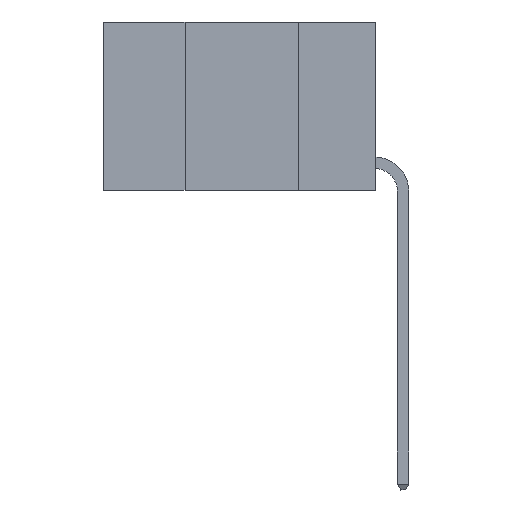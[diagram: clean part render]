
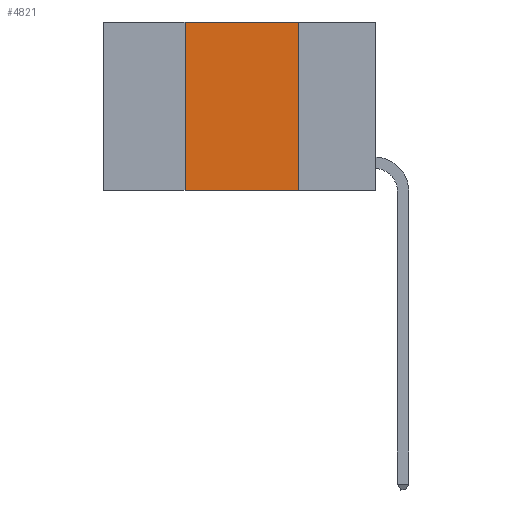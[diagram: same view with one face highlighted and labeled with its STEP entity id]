
A CAD part, left-side view. The second image highlights one B-rep face of the part: STEP entity #4821.
In plain terms, the highlighted planar face has unit normal (-1, 0, 0).
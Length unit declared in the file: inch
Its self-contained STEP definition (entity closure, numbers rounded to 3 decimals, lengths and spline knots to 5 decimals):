
#1 = DIRECTION ( 'NONE',  ( 0., 0., 1. ) ) ;
#532 = VECTOR ( 'NONE', #12277, 39.37008 ) ;
#628 = ORIENTED_EDGE ( 'NONE', *, *, #4704, .F. ) ;
#1104 = DIRECTION ( 'NONE',  ( 0., -1., 0. ) ) ;
#1490 = VERTEX_POINT ( 'NONE', #5422 ) ;
#1825 = VERTEX_POINT ( 'NONE', #3805 ) ;
#1961 = VERTEX_POINT ( 'NONE', #15304 ) ;
#2581 = ORIENTED_EDGE ( 'NONE', *, *, #4188, .F. ) ;
#2772 = DIRECTION ( 'NONE',  ( 1., 0., 0. ) ) ;
#3540 = CARTESIAN_POINT ( 'NONE',  ( 0., 0.17, 0. ) ) ;
#3805 = CARTESIAN_POINT ( 'NONE',  ( 0., 0.42, 0. ) ) ;
#4188 = EDGE_CURVE ( 'NONE', #1825, #1961, #5525, .T. ) ;
#4704 = EDGE_CURVE ( 'NONE', #1961, #10951, #6226, .T. ) ;
#4821 = ADVANCED_FACE ( 'NONE', ( #10494 ), #7730, .F. ) ;
#5422 = CARTESIAN_POINT ( 'NONE',  ( 0., 0.42, -0.37 ) ) ;
#5525 = LINE ( 'NONE', #9837, #532 ) ;
#6067 = CARTESIAN_POINT ( 'NONE',  ( 0., 0.6, -0.37 ) ) ;
#6226 = LINE ( 'NONE', #3540, #11155 ) ;
#7207 = VECTOR ( 'NONE', #1104, 39.37008 ) ;
#7730 = PLANE ( 'NONE',  #14382 ) ;
#8379 = ORIENTED_EDGE ( 'NONE', *, *, #8780, .T. ) ;
#8780 = EDGE_CURVE ( 'NONE', #1490, #10951, #11082, .T. ) ;
#8816 = LINE ( 'NONE', #13757, #12659 ) ;
#8992 = CARTESIAN_POINT ( 'NONE',  ( 0., 0.17, -0.37 ) ) ;
#9814 = DIRECTION ( 'NONE',  ( 0., 0., -1. ) ) ;
#9837 = CARTESIAN_POINT ( 'NONE',  ( 0., 0.6, 0. ) ) ;
#10494 = FACE_OUTER_BOUND ( 'NONE', #12740, .T. ) ;
#10951 = VERTEX_POINT ( 'NONE', #8992 ) ;
#11082 = LINE ( 'NONE', #6067, #7207 ) ;
#11155 = VECTOR ( 'NONE', #9814, 39.37008 ) ;
#12277 = DIRECTION ( 'NONE',  ( 0., -1., 0. ) ) ;
#12659 = VECTOR ( 'NONE', #1, 39.37008 ) ;
#12740 = EDGE_LOOP ( 'NONE', ( #628, #2581, #13568, #8379 ) ) ;
#12789 = EDGE_CURVE ( 'NONE', #1490, #1825, #8816, .T. ) ;
#13568 = ORIENTED_EDGE ( 'NONE', *, *, #12789, .F. ) ;
#13757 = CARTESIAN_POINT ( 'NONE',  ( 0., 0.42, 0. ) ) ;
#14382 = AXIS2_PLACEMENT_3D ( 'NONE', #15542, #2772, #15693 ) ;
#15304 = CARTESIAN_POINT ( 'NONE',  ( 0., 0.17, 0. ) ) ;
#15542 = CARTESIAN_POINT ( 'NONE',  ( 0., 0.6, 0. ) ) ;
#15693 = DIRECTION ( 'NONE',  ( 0., 0., -1. ) ) ;
